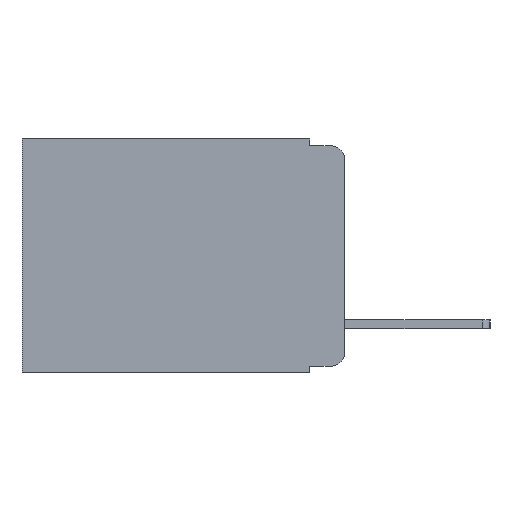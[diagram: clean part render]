
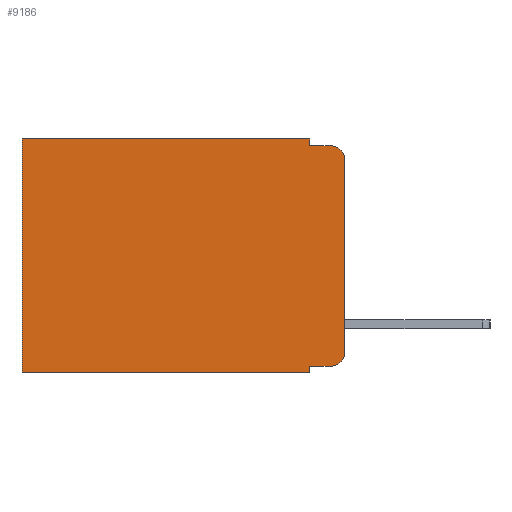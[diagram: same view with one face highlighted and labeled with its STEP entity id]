
A CAD part, left-side view. The second image highlights one B-rep face of the part: STEP entity #9186.
In plain terms, the highlighted planar face has unit normal (-1, 0, 0).
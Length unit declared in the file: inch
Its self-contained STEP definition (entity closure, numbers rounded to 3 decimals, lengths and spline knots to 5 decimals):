
#190 = ORIENTED_EDGE ( 'NONE', *, *, #2300, .F. ) ;
#686 = CARTESIAN_POINT ( 'NONE',  ( 0.298, 0., 0. ) ) ;
#764 = DIRECTION ( 'NONE',  ( 0., 0., -1. ) ) ;
#904 = CARTESIAN_POINT ( 'NONE',  ( 0.298, 0.051, 0. ) ) ;
#1128 = DIRECTION ( 'NONE',  ( -1., 0., 0. ) ) ;
#1140 = LINE ( 'NONE', #10661, #14279 ) ;
#1213 = VECTOR ( 'NONE', #4526, 39.37008 ) ;
#1538 = AXIS2_PLACEMENT_3D ( 'NONE', #7144, #12134, #4501 ) ;
#1542 = CARTESIAN_POINT ( 'NONE',  ( 0.298, 0.051, -0.333 ) ) ;
#1554 = DIRECTION ( 'NONE',  ( 0., 0., -1. ) ) ;
#1781 = VERTEX_POINT ( 'NONE', #9474 ) ;
#1795 = VECTOR ( 'NONE', #6995, 39.37008 ) ;
#2300 = EDGE_CURVE ( 'NONE', #10871, #3316, #15208, .T. ) ;
#2371 = EDGE_CURVE ( 'NONE', #4580, #1781, #14082, .T. ) ;
#2672 = CARTESIAN_POINT ( 'NONE',  ( 0.298, 0.051, -0.333 ) ) ;
#3082 = FACE_OUTER_BOUND ( 'NONE', #5458, .T. ) ;
#3125 = CARTESIAN_POINT ( 'NONE',  ( 0.298, 0.02, -0.333 ) ) ;
#3316 = VERTEX_POINT ( 'NONE', #5243 ) ;
#3664 = VECTOR ( 'NONE', #764, 39.37008 ) ;
#3888 = LINE ( 'NONE', #686, #7425 ) ;
#3920 = VECTOR ( 'NONE', #1554, 39.37008 ) ;
#3971 = DIRECTION ( 'NONE',  ( 0., -1., 0. ) ) ;
#4233 = DIRECTION ( 'NONE',  ( 0., 1., 0. ) ) ;
#4501 = DIRECTION ( 'NONE',  ( 0., 0., -1. ) ) ;
#4526 = DIRECTION ( 'NONE',  ( 0., 0., -1. ) ) ;
#4580 = VERTEX_POINT ( 'NONE', #1542 ) ;
#4706 = VERTEX_POINT ( 'NONE', #13597 ) ;
#4829 = VERTEX_POINT ( 'NONE', #15165 ) ;
#5243 = CARTESIAN_POINT ( 'NONE',  ( 0.298, 0.02, -0.01 ) ) ;
#5458 = EDGE_LOOP ( 'NONE', ( #11074, #12053, #190, #15190, #9924, #12419, #6346, #9736, #6154, #10120 ) ) ;
#5849 = DIRECTION ( 'NONE',  ( -1., 0., 0. ) ) ;
#6154 = ORIENTED_EDGE ( 'NONE', *, *, #8185, .T. ) ;
#6207 = VECTOR ( 'NONE', #3971, 39.37008 ) ;
#6346 = ORIENTED_EDGE ( 'NONE', *, *, #9056, .F. ) ;
#6872 = CARTESIAN_POINT ( 'NONE',  ( 0.298, 0.051, 0. ) ) ;
#6995 = DIRECTION ( 'NONE',  ( 0., -1., 0. ) ) ;
#7121 = CARTESIAN_POINT ( 'NONE',  ( 0.298, 0., 0. ) ) ;
#7144 = CARTESIAN_POINT ( 'NONE',  ( 0.298, 0., 0. ) ) ;
#7297 = EDGE_CURVE ( 'NONE', #4829, #4706, #14340, .T. ) ;
#7375 = DIRECTION ( 'NONE',  ( 0., 0., -1. ) ) ;
#7425 = VECTOR ( 'NONE', #7375, 39.37008 ) ;
#7469 = CARTESIAN_POINT ( 'NONE',  ( 0.298, 0.051, -0.01 ) ) ;
#7549 = VERTEX_POINT ( 'NONE', #9071 ) ;
#7728 = EDGE_CURVE ( 'NONE', #13183, #10871, #7879, .T. ) ;
#7879 = LINE ( 'NONE', #6872, #3920 ) ;
#7962 = CARTESIAN_POINT ( 'NONE',  ( 0.298, 0.051, 0. ) ) ;
#8071 = CIRCLE ( 'NONE', #14122, 0.02 ) ;
#8178 = LINE ( 'NONE', #7121, #11059 ) ;
#8185 = EDGE_CURVE ( 'NONE', #4580, #10826, #15967, .T. ) ;
#8598 = EDGE_CURVE ( 'NONE', #11033, #7549, #3888, .T. ) ;
#9023 = CARTESIAN_POINT ( 'NONE',  ( 0.298, 0.02, -0.313 ) ) ;
#9056 = EDGE_CURVE ( 'NONE', #1781, #4706, #1140, .T. ) ;
#9071 = CARTESIAN_POINT ( 'NONE',  ( 0.298, 0., -0.313 ) ) ;
#9186 = ADVANCED_FACE ( 'NONE', ( #3082 ), #10916, .F. ) ;
#9474 = CARTESIAN_POINT ( 'NONE',  ( 0.298, 0.051, -0.343 ) ) ;
#9703 = CIRCLE ( 'NONE', #12820, 0.02 ) ;
#9736 = ORIENTED_EDGE ( 'NONE', *, *, #2371, .F. ) ;
#9924 = ORIENTED_EDGE ( 'NONE', *, *, #10822, .T. ) ;
#10120 = ORIENTED_EDGE ( 'NONE', *, *, #11147, .T. ) ;
#10295 = DIRECTION ( 'NONE',  ( 0., 0., -1. ) ) ;
#10661 = CARTESIAN_POINT ( 'NONE',  ( 0.298, 0., -0.343 ) ) ;
#10822 = EDGE_CURVE ( 'NONE', #13183, #4829, #8178, .T. ) ;
#10826 = VERTEX_POINT ( 'NONE', #3125 ) ;
#10871 = VERTEX_POINT ( 'NONE', #13337 ) ;
#10916 = PLANE ( 'NONE',  #1538 ) ;
#11033 = VERTEX_POINT ( 'NONE', #13572 ) ;
#11059 = VECTOR ( 'NONE', #15619, 39.37008 ) ;
#11074 = ORIENTED_EDGE ( 'NONE', *, *, #8598, .F. ) ;
#11147 = EDGE_CURVE ( 'NONE', #10826, #7549, #9703, .T. ) ;
#12053 = ORIENTED_EDGE ( 'NONE', *, *, #15689, .T. ) ;
#12134 = DIRECTION ( 'NONE',  ( 1., 0., 0. ) ) ;
#12419 = ORIENTED_EDGE ( 'NONE', *, *, #7297, .T. ) ;
#12820 = AXIS2_PLACEMENT_3D ( 'NONE', #9023, #1128, #10295 ) ;
#13183 = VERTEX_POINT ( 'NONE', #904 ) ;
#13311 = CARTESIAN_POINT ( 'NONE',  ( 0.298, 0.02, -0.03 ) ) ;
#13327 = CARTESIAN_POINT ( 'NONE',  ( 0.298, 0.473, 0. ) ) ;
#13337 = CARTESIAN_POINT ( 'NONE',  ( 0.298, 0.051, -0.01 ) ) ;
#13572 = CARTESIAN_POINT ( 'NONE',  ( 0.298, 0., -0.03 ) ) ;
#13597 = CARTESIAN_POINT ( 'NONE',  ( 0.298, 0.473, -0.343 ) ) ;
#14082 = LINE ( 'NONE', #7962, #3664 ) ;
#14122 = AXIS2_PLACEMENT_3D ( 'NONE', #13311, #5849, #14508 ) ;
#14279 = VECTOR ( 'NONE', #4233, 39.37008 ) ;
#14340 = LINE ( 'NONE', #13327, #1213 ) ;
#14508 = DIRECTION ( 'NONE',  ( 0., 0., -1. ) ) ;
#15165 = CARTESIAN_POINT ( 'NONE',  ( 0.298, 0.473, 0. ) ) ;
#15190 = ORIENTED_EDGE ( 'NONE', *, *, #7728, .F. ) ;
#15208 = LINE ( 'NONE', #7469, #1795 ) ;
#15619 = DIRECTION ( 'NONE',  ( 0., 1., 0. ) ) ;
#15689 = EDGE_CURVE ( 'NONE', #11033, #3316, #8071, .T. ) ;
#15967 = LINE ( 'NONE', #2672, #6207 ) ;
